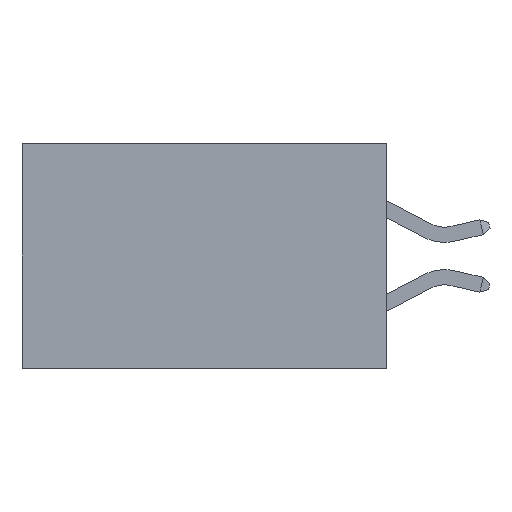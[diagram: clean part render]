
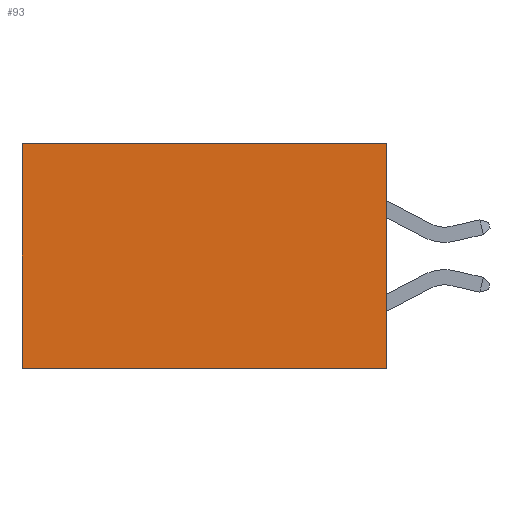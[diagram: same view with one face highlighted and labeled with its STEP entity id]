
A CAD part, left-side view. The second image highlights one B-rep face of the part: STEP entity #93.
In plain terms, the highlighted planar face has unit normal (-1, 0, 0).
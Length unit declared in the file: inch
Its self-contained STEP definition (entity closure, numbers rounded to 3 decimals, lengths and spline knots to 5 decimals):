
#93 = ADVANCED_FACE ( 'NONE', ( #121 ), #1580, .F. ) ;
#121 = FACE_OUTER_BOUND ( 'NONE', #14626, .T. ) ;
#645 = ORIENTED_EDGE ( 'NONE', *, *, #13472, .T. ) ;
#1580 = PLANE ( 'NONE',  #7205 ) ;
#3010 = EDGE_CURVE ( 'NONE', #16012, #17372, #6103, .T. ) ;
#3806 = CARTESIAN_POINT ( 'NONE',  ( 0.298, 0., 0. ) ) ;
#4877 = EDGE_CURVE ( 'NONE', #8621, #16012, #24802, .T. ) ;
#5672 = DIRECTION ( 'NONE',  ( 0., 1., 0. ) ) ;
#6103 = LINE ( 'NONE', #12910, #20843 ) ;
#6977 = DIRECTION ( 'NONE',  ( 0., 0., -1. ) ) ;
#7031 = CARTESIAN_POINT ( 'NONE',  ( 0.298, 0., 0. ) ) ;
#7205 = AXIS2_PLACEMENT_3D ( 'NONE', #22275, #25589, #25740 ) ;
#7588 = VECTOR ( 'NONE', #5672, 39.37008 ) ;
#8230 = LINE ( 'NONE', #15751, #7588 ) ;
#8621 = VERTEX_POINT ( 'NONE', #3806 ) ;
#9282 = LINE ( 'NONE', #14403, #18701 ) ;
#12278 = CARTESIAN_POINT ( 'NONE',  ( 0.298, 0.6, 0. ) ) ;
#12504 = CARTESIAN_POINT ( 'NONE',  ( 0.298, 0., -0.37 ) ) ;
#12910 = CARTESIAN_POINT ( 'NONE',  ( 0.298, 0., -0.37 ) ) ;
#13472 = EDGE_CURVE ( 'NONE', #15216, #17372, #9282, .T. ) ;
#14403 = CARTESIAN_POINT ( 'NONE',  ( 0.298, 0.6, 0. ) ) ;
#14626 = EDGE_LOOP ( 'NONE', ( #645, #20802, #17432, #20004 ) ) ;
#15216 = VERTEX_POINT ( 'NONE', #12278 ) ;
#15392 = DIRECTION ( 'NONE',  ( 0., 1., 0. ) ) ;
#15751 = CARTESIAN_POINT ( 'NONE',  ( 0.298, 0., 0. ) ) ;
#16012 = VERTEX_POINT ( 'NONE', #12504 ) ;
#17372 = VERTEX_POINT ( 'NONE', #18870 ) ;
#17432 = ORIENTED_EDGE ( 'NONE', *, *, #4877, .F. ) ;
#17678 = EDGE_CURVE ( 'NONE', #8621, #15216, #8230, .T. ) ;
#18701 = VECTOR ( 'NONE', #20379, 39.37008 ) ;
#18870 = CARTESIAN_POINT ( 'NONE',  ( 0.298, 0.6, -0.37 ) ) ;
#20004 = ORIENTED_EDGE ( 'NONE', *, *, #17678, .T. ) ;
#20379 = DIRECTION ( 'NONE',  ( 0., 0., -1. ) ) ;
#20802 = ORIENTED_EDGE ( 'NONE', *, *, #3010, .F. ) ;
#20843 = VECTOR ( 'NONE', #15392, 39.37008 ) ;
#22275 = CARTESIAN_POINT ( 'NONE',  ( 0.298, 0., 0. ) ) ;
#24802 = LINE ( 'NONE', #7031, #25422 ) ;
#25422 = VECTOR ( 'NONE', #6977, 39.37008 ) ;
#25589 = DIRECTION ( 'NONE',  ( 1., 0., 0. ) ) ;
#25740 = DIRECTION ( 'NONE',  ( 0., 0., -1. ) ) ;
